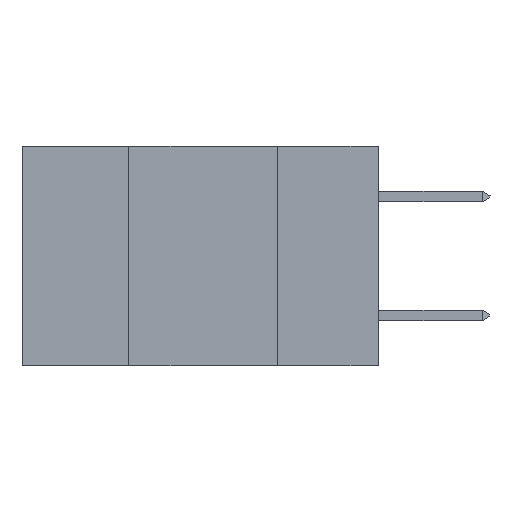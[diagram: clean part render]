
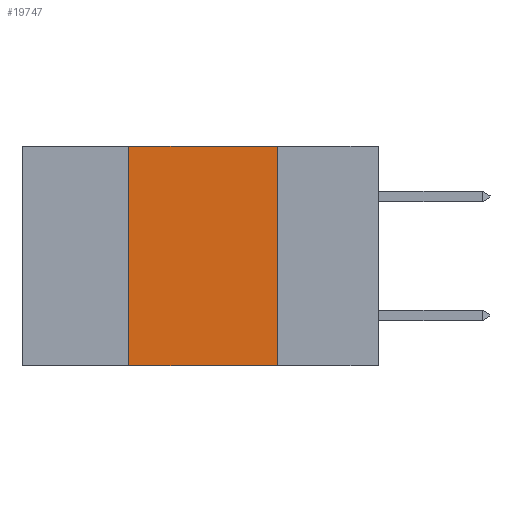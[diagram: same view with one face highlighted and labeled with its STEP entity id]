
A CAD part, left-side view. The second image highlights one B-rep face of the part: STEP entity #19747.
In plain terms, the highlighted planar face has unit normal (-1, 0, 0).
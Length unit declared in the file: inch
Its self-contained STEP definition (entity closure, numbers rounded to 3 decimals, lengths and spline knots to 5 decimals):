
#451 = DIRECTION ( 'NONE',  ( 0., 0., -1. ) ) ;
#1012 = DIRECTION ( 'NONE',  ( 0., -1., 0. ) ) ;
#2070 = VERTEX_POINT ( 'NONE', #9211 ) ;
#2713 = ORIENTED_EDGE ( 'NONE', *, *, #5230, .F. ) ;
#3126 = VECTOR ( 'NONE', #20111, 39.37008 ) ;
#3150 = EDGE_LOOP ( 'NONE', ( #2713, #3400, #15115, #12778 ) ) ;
#3239 = VERTEX_POINT ( 'NONE', #9382 ) ;
#3400 = ORIENTED_EDGE ( 'NONE', *, *, #18979, .F. ) ;
#3896 = CARTESIAN_POINT ( 'NONE',  ( 0., 0.6, 0. ) ) ;
#4321 = EDGE_CURVE ( 'NONE', #2070, #15145, #11358, .T. ) ;
#4585 = VERTEX_POINT ( 'NONE', #13394 ) ;
#5230 = EDGE_CURVE ( 'NONE', #3239, #15145, #8657, .T. ) ;
#6585 = CARTESIAN_POINT ( 'NONE',  ( 0., 0.42, -0.37 ) ) ;
#6602 = LINE ( 'NONE', #21846, #3126 ) ;
#6900 = EDGE_CURVE ( 'NONE', #2070, #4585, #11641, .T. ) ;
#7575 = AXIS2_PLACEMENT_3D ( 'NONE', #3896, #9200, #451 ) ;
#8271 = CARTESIAN_POINT ( 'NONE',  ( 0., 0.6, -0.37 ) ) ;
#8657 = LINE ( 'NONE', #20678, #13589 ) ;
#9200 = DIRECTION ( 'NONE',  ( 1., 0., 0. ) ) ;
#9211 = CARTESIAN_POINT ( 'NONE',  ( 0., 0.42, -0.37 ) ) ;
#9382 = CARTESIAN_POINT ( 'NONE',  ( 0., 0.17, 0. ) ) ;
#9396 = VECTOR ( 'NONE', #22641, 39.37008 ) ;
#11358 = LINE ( 'NONE', #8271, #17911 ) ;
#11641 = LINE ( 'NONE', #6585, #9396 ) ;
#12196 = DIRECTION ( 'NONE',  ( 0., 0., -1. ) ) ;
#12625 = PLANE ( 'NONE',  #7575 ) ;
#12778 = ORIENTED_EDGE ( 'NONE', *, *, #4321, .T. ) ;
#13394 = CARTESIAN_POINT ( 'NONE',  ( 0., 0.42, 0. ) ) ;
#13589 = VECTOR ( 'NONE', #12196, 39.37008 ) ;
#15115 = ORIENTED_EDGE ( 'NONE', *, *, #6900, .F. ) ;
#15145 = VERTEX_POINT ( 'NONE', #19965 ) ;
#17911 = VECTOR ( 'NONE', #1012, 39.37008 ) ;
#18979 = EDGE_CURVE ( 'NONE', #4585, #3239, #6602, .T. ) ;
#19747 = ADVANCED_FACE ( 'NONE', ( #21325 ), #12625, .F. ) ;
#19965 = CARTESIAN_POINT ( 'NONE',  ( 0., 0.17, -0.37 ) ) ;
#20111 = DIRECTION ( 'NONE',  ( 0., -1., 0. ) ) ;
#20678 = CARTESIAN_POINT ( 'NONE',  ( 0., 0.17, -0.37 ) ) ;
#21325 = FACE_OUTER_BOUND ( 'NONE', #3150, .T. ) ;
#21846 = CARTESIAN_POINT ( 'NONE',  ( 0., 0.6, 0. ) ) ;
#22641 = DIRECTION ( 'NONE',  ( 0., 0., 1. ) ) ;
